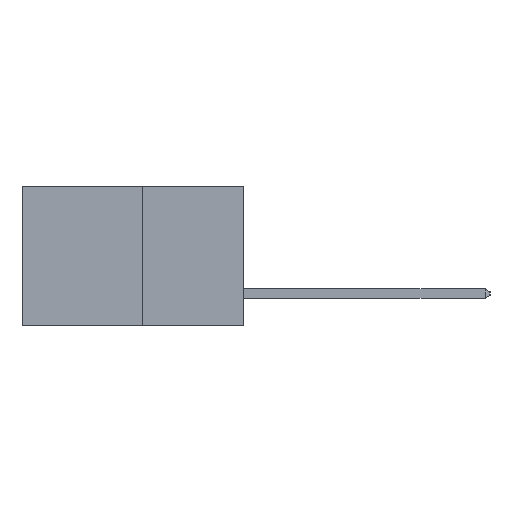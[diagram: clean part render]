
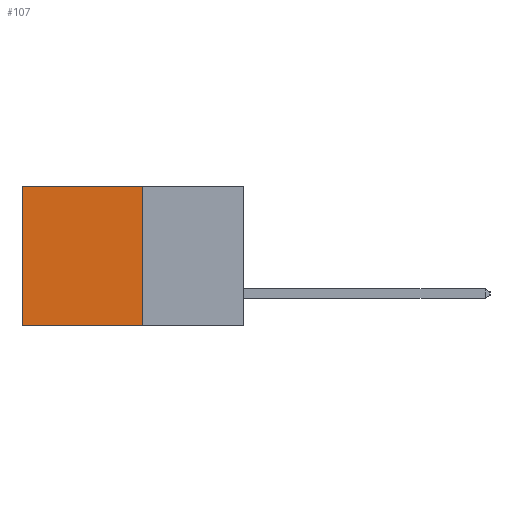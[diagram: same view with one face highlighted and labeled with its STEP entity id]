
A CAD part, left-side view. The second image highlights one B-rep face of the part: STEP entity #107.
In plain terms, the highlighted planar face has unit normal (-1, 0, 0).
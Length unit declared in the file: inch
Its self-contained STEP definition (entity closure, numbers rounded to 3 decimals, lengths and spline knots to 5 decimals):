
#35 = CARTESIAN_POINT ( 'NONE',  ( 0.277, 0.59, 0. ) ) ;
#107 = ADVANCED_FACE ( 'NONE', ( #687 ), #1342, .F. ) ;
#672 = CARTESIAN_POINT ( 'NONE',  ( 0.277, 0.27, 0. ) ) ;
#687 = FACE_OUTER_BOUND ( 'NONE', #16170, .T. ) ;
#1342 = PLANE ( 'NONE',  #14828 ) ;
#1732 = DIRECTION ( 'NONE',  ( 0., 1., 0. ) ) ;
#2641 = VECTOR ( 'NONE', #12298, 39.37008 ) ;
#3066 = EDGE_CURVE ( 'NONE', #13077, #14740, #22396, .T. ) ;
#3313 = ORIENTED_EDGE ( 'NONE', *, *, #3066, .T. ) ;
#3383 = VERTEX_POINT ( 'NONE', #672 ) ;
#3916 = EDGE_CURVE ( 'NONE', #9487, #14740, #18620, .T. ) ;
#5345 = EDGE_CURVE ( 'NONE', #3383, #9487, #16062, .T. ) ;
#7700 = CARTESIAN_POINT ( 'NONE',  ( 0.277, 0.27, 0. ) ) ;
#7927 = ORIENTED_EDGE ( 'NONE', *, *, #21181, .T. ) ;
#8311 = CARTESIAN_POINT ( 'NONE',  ( 0.277, 0.27, -0.37 ) ) ;
#9487 = VERTEX_POINT ( 'NONE', #8311 ) ;
#10155 = DIRECTION ( 'NONE',  ( 1., 0., 0. ) ) ;
#10224 = VECTOR ( 'NONE', #1732, 39.37008 ) ;
#10313 = CARTESIAN_POINT ( 'NONE',  ( 0.277, 0.27, -0.37 ) ) ;
#10666 = DIRECTION ( 'NONE',  ( 0., 0., -1. ) ) ;
#11562 = CARTESIAN_POINT ( 'NONE',  ( 0.277, 0.59, -0.37 ) ) ;
#12298 = DIRECTION ( 'NONE',  ( 0., 1., 0. ) ) ;
#12486 = ORIENTED_EDGE ( 'NONE', *, *, #5345, .F. ) ;
#13077 = VERTEX_POINT ( 'NONE', #35 ) ;
#14740 = VERTEX_POINT ( 'NONE', #25519 ) ;
#14828 = AXIS2_PLACEMENT_3D ( 'NONE', #24695, #10155, #19362 ) ;
#16062 = LINE ( 'NONE', #20598, #25311 ) ;
#16169 = LINE ( 'NONE', #7700, #10224 ) ;
#16170 = EDGE_LOOP ( 'NONE', ( #3313, #22931, #12486, #7927 ) ) ;
#18620 = LINE ( 'NONE', #10313, #2641 ) ;
#19362 = DIRECTION ( 'NONE',  ( 0., 0., -1. ) ) ;
#20598 = CARTESIAN_POINT ( 'NONE',  ( 0.277, 0.27, -0.37 ) ) ;
#21181 = EDGE_CURVE ( 'NONE', #3383, #13077, #16169, .T. ) ;
#22396 = LINE ( 'NONE', #11562, #22921 ) ;
#22921 = VECTOR ( 'NONE', #23470, 39.37008 ) ;
#22931 = ORIENTED_EDGE ( 'NONE', *, *, #3916, .F. ) ;
#23470 = DIRECTION ( 'NONE',  ( 0., 0., -1. ) ) ;
#24695 = CARTESIAN_POINT ( 'NONE',  ( 0.277, 0.27, -0.37 ) ) ;
#25311 = VECTOR ( 'NONE', #10666, 39.37008 ) ;
#25519 = CARTESIAN_POINT ( 'NONE',  ( 0.277, 0.59, -0.37 ) ) ;
